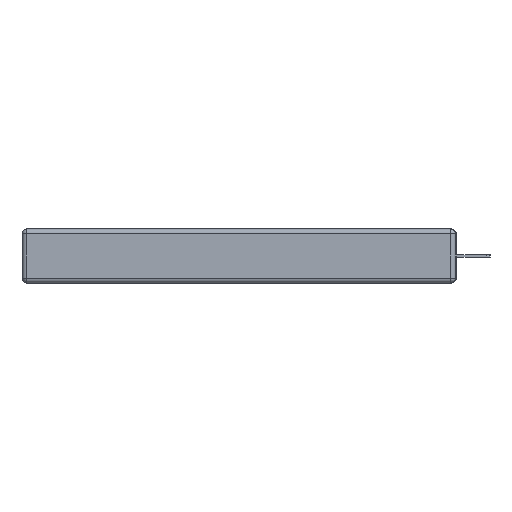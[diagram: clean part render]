
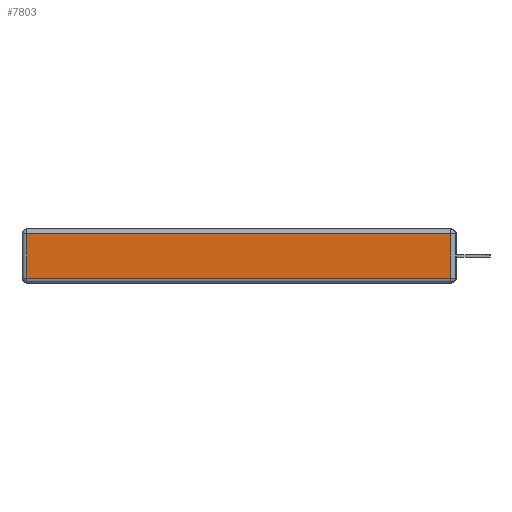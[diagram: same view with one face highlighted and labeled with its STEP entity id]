
A CAD part, left-side view. The second image highlights one B-rep face of the part: STEP entity #7803.
In plain terms, the highlighted planar face has unit normal (-1, 0, 0).
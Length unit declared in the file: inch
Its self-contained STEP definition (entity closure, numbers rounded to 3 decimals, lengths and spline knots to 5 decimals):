
#1427 = ORIENTED_EDGE ( 'NONE', *, *, #19778, .T. ) ;
#1515 = VECTOR ( 'NONE', #22133, 39.37008 ) ;
#2008 = DIRECTION ( 'NONE',  ( 0., 1., 0. ) ) ;
#2322 = ORIENTED_EDGE ( 'NONE', *, *, #6243, .T. ) ;
#4911 = DIRECTION ( 'NONE',  ( -1., 0., 0. ) ) ;
#6133 = EDGE_LOOP ( 'NONE', ( #2322, #1427, #24846, #25365 ) ) ;
#6243 = EDGE_CURVE ( 'NONE', #9587, #9913, #19747, .T. ) ;
#7246 = CARTESIAN_POINT ( 'NONE',  ( 0., 0., -0.343 ) ) ;
#7658 = EDGE_CURVE ( 'NONE', #9830, #9587, #24471, .T. ) ;
#7803 = ADVANCED_FACE ( 'NONE', ( #27506 ), #9910, .T. ) ;
#8424 = EDGE_CURVE ( 'NONE', #11593, #9830, #10013, .T. ) ;
#9053 = CARTESIAN_POINT ( 'NONE',  ( 0., 2.72, -0.343 ) ) ;
#9587 = VERTEX_POINT ( 'NONE', #26863 ) ;
#9830 = VERTEX_POINT ( 'NONE', #16724 ) ;
#9910 = PLANE ( 'NONE',  #13737 ) ;
#9913 = VERTEX_POINT ( 'NONE', #15114 ) ;
#10013 = LINE ( 'NONE', #21889, #18897 ) ;
#10952 = DIRECTION ( 'NONE',  ( 0., -1., 0. ) ) ;
#11593 = VERTEX_POINT ( 'NONE', #12216 ) ;
#12216 = CARTESIAN_POINT ( 'NONE',  ( 0., 0.03, -0.03 ) ) ;
#12735 = VECTOR ( 'NONE', #10952, 39.37008 ) ;
#13737 = AXIS2_PLACEMENT_3D ( 'NONE', #7246, #4911, #16080 ) ;
#14219 = CARTESIAN_POINT ( 'NONE',  ( 0., 0.03, -0.343 ) ) ;
#15114 = CARTESIAN_POINT ( 'NONE',  ( 0., 0.03, -0.313 ) ) ;
#16080 = DIRECTION ( 'NONE',  ( 0., 0., 1. ) ) ;
#16406 = DIRECTION ( 'NONE',  ( 0., 0., 1. ) ) ;
#16724 = CARTESIAN_POINT ( 'NONE',  ( 0., 2.72, -0.03 ) ) ;
#17618 = VECTOR ( 'NONE', #16406, 39.37008 ) ;
#18897 = VECTOR ( 'NONE', #2008, 39.37008 ) ;
#19747 = LINE ( 'NONE', #22106, #12735 ) ;
#19778 = EDGE_CURVE ( 'NONE', #9913, #11593, #27546, .T. ) ;
#21889 = CARTESIAN_POINT ( 'NONE',  ( 0., 2.75, -0.03 ) ) ;
#22106 = CARTESIAN_POINT ( 'NONE',  ( 0., 0., -0.313 ) ) ;
#22133 = DIRECTION ( 'NONE',  ( 0., 0., -1. ) ) ;
#24471 = LINE ( 'NONE', #9053, #1515 ) ;
#24846 = ORIENTED_EDGE ( 'NONE', *, *, #8424, .T. ) ;
#25365 = ORIENTED_EDGE ( 'NONE', *, *, #7658, .T. ) ;
#26863 = CARTESIAN_POINT ( 'NONE',  ( 0., 2.72, -0.313 ) ) ;
#27506 = FACE_OUTER_BOUND ( 'NONE', #6133, .T. ) ;
#27546 = LINE ( 'NONE', #14219, #17618 ) ;
